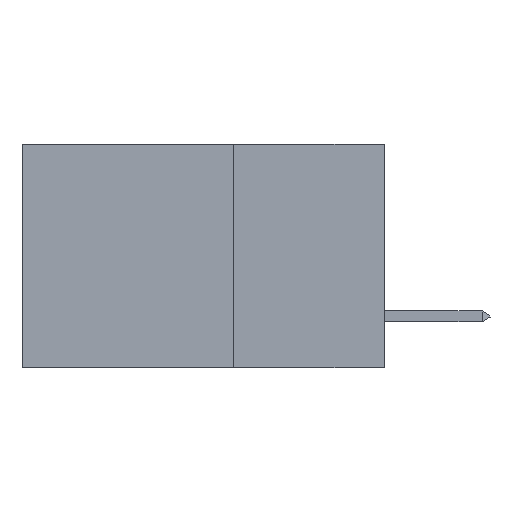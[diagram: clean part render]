
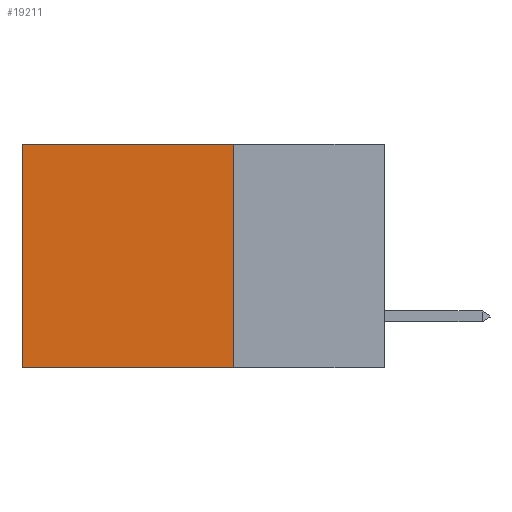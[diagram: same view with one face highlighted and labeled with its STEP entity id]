
A CAD part, left-side view. The second image highlights one B-rep face of the part: STEP entity #19211.
In plain terms, the highlighted planar face has unit normal (-1, 0, 0).
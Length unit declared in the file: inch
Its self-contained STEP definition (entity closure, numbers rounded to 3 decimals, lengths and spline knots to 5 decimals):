
#483 = EDGE_CURVE ( 'NONE', #30444, #33727, #17661, .T. ) ;
#502 = CARTESIAN_POINT ( 'NONE',  ( 0.2875, 0.25, 0. ) ) ;
#974 = CARTESIAN_POINT ( 'NONE',  ( 0.2875, 0.25, 0. ) ) ;
#3070 = VECTOR ( 'NONE', #10522, 39.37008 ) ;
#4317 = DIRECTION ( 'NONE',  ( 0., 1., 0. ) ) ;
#5083 = VECTOR ( 'NONE', #17612, 39.37008 ) ;
#7878 = ORIENTED_EDGE ( 'NONE', *, *, #483, .T. ) ;
#7956 = PLANE ( 'NONE',  #12115 ) ;
#8359 = CARTESIAN_POINT ( 'NONE',  ( 0.2875, 0.6, -0.37 ) ) ;
#10273 = CARTESIAN_POINT ( 'NONE',  ( 0.2875, 0.6, 0. ) ) ;
#10522 = DIRECTION ( 'NONE',  ( 0., 0., -1. ) ) ;
#12115 = AXIS2_PLACEMENT_3D ( 'NONE', #16619, #33564, #30781 ) ;
#12382 = ORIENTED_EDGE ( 'NONE', *, *, #16282, .F. ) ;
#13858 = LINE ( 'NONE', #10273, #3070 ) ;
#15457 = ORIENTED_EDGE ( 'NONE', *, *, #20053, .T. ) ;
#15729 = CARTESIAN_POINT ( 'NONE',  ( 0.2875, 0.25, -0.37 ) ) ;
#15822 = VECTOR ( 'NONE', #4317, 39.37008 ) ;
#16282 = EDGE_CURVE ( 'NONE', #30444, #21179, #35629, .T. ) ;
#16320 = EDGE_LOOP ( 'NONE', ( #15457, #20780, #12382, #7878 ) ) ;
#16619 = CARTESIAN_POINT ( 'NONE',  ( 0.2875, 0.25, 0. ) ) ;
#17612 = DIRECTION ( 'NONE',  ( 0., 0., -1. ) ) ;
#17661 = LINE ( 'NONE', #974, #27543 ) ;
#19211 = ADVANCED_FACE ( 'NONE', ( #26932 ), #7956, .F. ) ;
#20053 = EDGE_CURVE ( 'NONE', #33727, #31951, #13858, .T. ) ;
#20780 = ORIENTED_EDGE ( 'NONE', *, *, #35102, .F. ) ;
#20883 = CARTESIAN_POINT ( 'NONE',  ( 0.2875, 0.25, -0.37 ) ) ;
#21179 = VERTEX_POINT ( 'NONE', #20883 ) ;
#21894 = CARTESIAN_POINT ( 'NONE',  ( 0.2875, 0.25, 0. ) ) ;
#23389 = CARTESIAN_POINT ( 'NONE',  ( 0.2875, 0.6, 0. ) ) ;
#26932 = FACE_OUTER_BOUND ( 'NONE', #16320, .T. ) ;
#27543 = VECTOR ( 'NONE', #35000, 39.37008 ) ;
#30444 = VERTEX_POINT ( 'NONE', #21894 ) ;
#30781 = DIRECTION ( 'NONE',  ( 0., 0., -1. ) ) ;
#31951 = VERTEX_POINT ( 'NONE', #8359 ) ;
#32418 = LINE ( 'NONE', #15729, #15822 ) ;
#33564 = DIRECTION ( 'NONE',  ( 1., 0., 0. ) ) ;
#33727 = VERTEX_POINT ( 'NONE', #23389 ) ;
#35000 = DIRECTION ( 'NONE',  ( 0., 1., 0. ) ) ;
#35102 = EDGE_CURVE ( 'NONE', #21179, #31951, #32418, .T. ) ;
#35629 = LINE ( 'NONE', #502, #5083 ) ;
